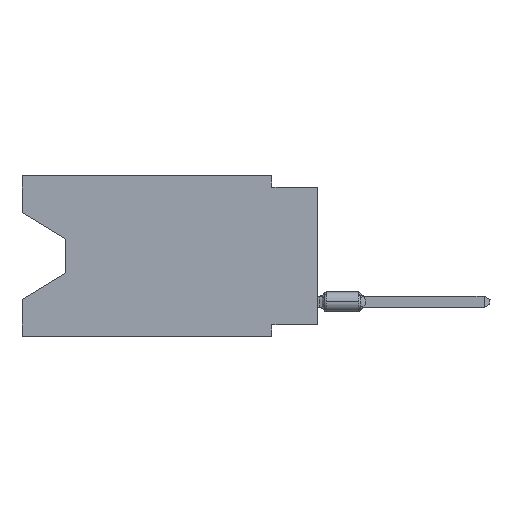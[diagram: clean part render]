
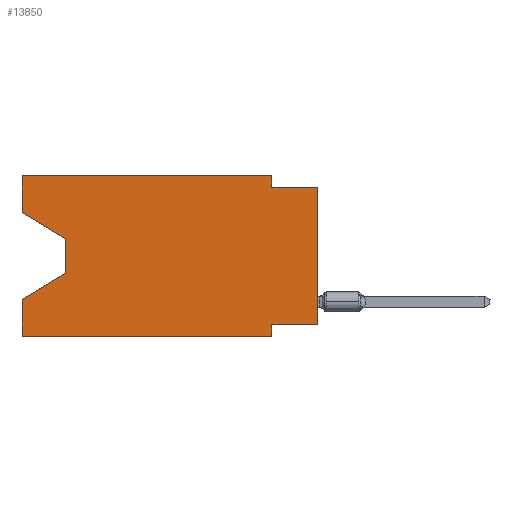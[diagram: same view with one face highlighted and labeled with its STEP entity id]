
A CAD part, left-side view. The second image highlights one B-rep face of the part: STEP entity #13850.
In plain terms, the highlighted planar face has unit normal (-1, 0, 0).
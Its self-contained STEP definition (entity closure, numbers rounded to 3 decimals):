
#352 = VECTOR ( 'NONE', #19690, 1000. ) ;
#1337 = VERTEX_POINT ( 'NONE', #20342 ) ;
#1892 = DIRECTION ( 'NONE',  ( 0., -1., 0. ) ) ;
#2032 = VECTOR ( 'NONE', #56872, 1000. ) ;
#2133 = CARTESIAN_POINT ( 'NONE',  ( 0., 0., -8.255 ) ) ;
#2474 = DIRECTION ( 'NONE',  ( 0., 0.855, -0.519 ) ) ;
#3121 = CARTESIAN_POINT ( 'NONE',  ( 0., 13.97, -5.385 ) ) ;
#4279 = EDGE_CURVE ( 'NONE', #62181, #1337, #60794, .T. ) ;
#5641 = ORIENTED_EDGE ( 'NONE', *, *, #9047, .T. ) ;
#7039 = CARTESIAN_POINT ( 'NONE',  ( 0., 0., 0. ) ) ;
#7942 = CARTESIAN_POINT ( 'NONE',  ( 0., 2.54, -0.635 ) ) ;
#8095 = ORIENTED_EDGE ( 'NONE', *, *, #42171, .F. ) ;
#8271 = ORIENTED_EDGE ( 'NONE', *, *, #28810, .F. ) ;
#8826 = VECTOR ( 'NONE', #18357, 1000. ) ;
#9047 = EDGE_CURVE ( 'NONE', #52611, #43932, #17225, .T. ) ;
#10908 = ORIENTED_EDGE ( 'NONE', *, *, #61993, .F. ) ;
#11304 = VERTEX_POINT ( 'NONE', #34492 ) ;
#11688 = DIRECTION ( 'NONE',  ( 0., -0.855, -0.519 ) ) ;
#13259 = LINE ( 'NONE', #28672, #27764 ) ;
#13850 = ADVANCED_FACE ( 'NONE', ( #31483 ), #57066, .F. ) ;
#14158 = ORIENTED_EDGE ( 'NONE', *, *, #15059, .T. ) ;
#14259 = VERTEX_POINT ( 'NONE', #31395 ) ;
#15059 = EDGE_CURVE ( 'NONE', #62181, #52611, #46918, .T. ) ;
#16546 = EDGE_CURVE ( 'NONE', #31232, #48138, #16653, .T. ) ;
#16595 = CARTESIAN_POINT ( 'NONE',  ( 0., 13.97, -3.505 ) ) ;
#16653 = LINE ( 'NONE', #7039, #27128 ) ;
#17225 = LINE ( 'NONE', #16595, #24915 ) ;
#17438 = DIRECTION ( 'NONE',  ( 0., 0., -1. ) ) ;
#17905 = LINE ( 'NONE', #32003, #44070 ) ;
#18357 = DIRECTION ( 'NONE',  ( 0., -1., 0. ) ) ;
#18675 = LINE ( 'NONE', #58027, #8826 ) ;
#19690 = DIRECTION ( 'NONE',  ( 0., -1., 0. ) ) ;
#20342 = CARTESIAN_POINT ( 'NONE',  ( 0., 16.383, 0. ) ) ;
#21467 = LINE ( 'NONE', #51500, #58059 ) ;
#22354 = CARTESIAN_POINT ( 'NONE',  ( 0., 16.383, -6.852 ) ) ;
#23044 = ORIENTED_EDGE ( 'NONE', *, *, #61592, .F. ) ;
#24915 = VECTOR ( 'NONE', #60155, 1000. ) ;
#26529 = VECTOR ( 'NONE', #50266, 1000. ) ;
#26585 = DIRECTION ( 'NONE',  ( 0., 0., 1. ) ) ;
#26794 = CARTESIAN_POINT ( 'NONE',  ( 0., 16.383, -2.038 ) ) ;
#27128 = VECTOR ( 'NONE', #46400, 1000. ) ;
#27764 = VECTOR ( 'NONE', #17438, 1000. ) ;
#28672 = CARTESIAN_POINT ( 'NONE',  ( 0., 2.54, -8.89 ) ) ;
#28810 = EDGE_CURVE ( 'NONE', #34464, #53646, #17905, .T. ) ;
#30456 = CARTESIAN_POINT ( 'NONE',  ( 0., 16.383, 0. ) ) ;
#31232 = VERTEX_POINT ( 'NONE', #36531 ) ;
#31395 = CARTESIAN_POINT ( 'NONE',  ( 0., 2.54, -8.255 ) ) ;
#31483 = FACE_OUTER_BOUND ( 'NONE', #56777, .T. ) ;
#32003 = CARTESIAN_POINT ( 'NONE',  ( 0., 2.54, 0. ) ) ;
#34364 = CARTESIAN_POINT ( 'NONE',  ( 0., 2.54, 0. ) ) ;
#34464 = VERTEX_POINT ( 'NONE', #34364 ) ;
#34492 = CARTESIAN_POINT ( 'NONE',  ( 0., 2.54, -8.89 ) ) ;
#35527 = LINE ( 'NONE', #40641, #45600 ) ;
#36531 = CARTESIAN_POINT ( 'NONE',  ( 0., 0., -8.255 ) ) ;
#37200 = DIRECTION ( 'NONE',  ( 1., 0., 0. ) ) ;
#37326 = LINE ( 'NONE', #2133, #2032 ) ;
#38382 = EDGE_CURVE ( 'NONE', #54183, #41645, #21467, .T. ) ;
#38821 = CARTESIAN_POINT ( 'NONE',  ( 0., 16.383, -8.89 ) ) ;
#38862 = LINE ( 'NONE', #58086, #352 ) ;
#39522 = CARTESIAN_POINT ( 'NONE',  ( 0., 13.97, -3.505 ) ) ;
#39587 = VECTOR ( 'NONE', #2474, 1000. ) ;
#40066 = ORIENTED_EDGE ( 'NONE', *, *, #4279, .F. ) ;
#40215 = VECTOR ( 'NONE', #11688, 1000. ) ;
#40641 = CARTESIAN_POINT ( 'NONE',  ( 0., 16.383, -8.89 ) ) ;
#41645 = VERTEX_POINT ( 'NONE', #22354 ) ;
#42004 = CARTESIAN_POINT ( 'NONE',  ( 0., 16.383, 0. ) ) ;
#42128 = AXIS2_PLACEMENT_3D ( 'NONE', #42004, #37200, #51305 ) ;
#42171 = EDGE_CURVE ( 'NONE', #1337, #34464, #38862, .T. ) ;
#43932 = VERTEX_POINT ( 'NONE', #52446 ) ;
#44070 = VECTOR ( 'NONE', #46385, 1000. ) ;
#44964 = EDGE_CURVE ( 'NONE', #54183, #11304, #35527, .T. ) ;
#45600 = VECTOR ( 'NONE', #1892, 1000. ) ;
#46385 = DIRECTION ( 'NONE',  ( 0., 0., -1. ) ) ;
#46400 = DIRECTION ( 'NONE',  ( 0., 0., 1. ) ) ;
#46878 = ORIENTED_EDGE ( 'NONE', *, *, #38382, .F. ) ;
#46918 = LINE ( 'NONE', #26794, #40215 ) ;
#48138 = VERTEX_POINT ( 'NONE', #56562 ) ;
#49716 = EDGE_CURVE ( 'NONE', #14259, #11304, #13259, .T. ) ;
#49773 = ORIENTED_EDGE ( 'NONE', *, *, #57723, .T. ) ;
#50266 = DIRECTION ( 'NONE',  ( 0., 0., 1. ) ) ;
#50386 = ORIENTED_EDGE ( 'NONE', *, *, #16546, .T. ) ;
#50832 = LINE ( 'NONE', #3121, #39587 ) ;
#51305 = DIRECTION ( 'NONE',  ( 0., 0., -1. ) ) ;
#51477 = ORIENTED_EDGE ( 'NONE', *, *, #49716, .F. ) ;
#51500 = CARTESIAN_POINT ( 'NONE',  ( 0., 16.383, 0. ) ) ;
#52150 = ORIENTED_EDGE ( 'NONE', *, *, #44964, .T. ) ;
#52446 = CARTESIAN_POINT ( 'NONE',  ( 0., 13.97, -5.385 ) ) ;
#52611 = VERTEX_POINT ( 'NONE', #39522 ) ;
#53646 = VERTEX_POINT ( 'NONE', #7942 ) ;
#53866 = CARTESIAN_POINT ( 'NONE',  ( 0., 16.383, -2.038 ) ) ;
#54183 = VERTEX_POINT ( 'NONE', #38821 ) ;
#56562 = CARTESIAN_POINT ( 'NONE',  ( 0., 0., -0.635 ) ) ;
#56777 = EDGE_LOOP ( 'NONE', ( #14158, #5641, #49773, #46878, #52150, #51477, #23044, #50386, #10908, #8271, #8095, #40066 ) ) ;
#56872 = DIRECTION ( 'NONE',  ( 0., 1., 0. ) ) ;
#57066 = PLANE ( 'NONE',  #42128 ) ;
#57723 = EDGE_CURVE ( 'NONE', #43932, #41645, #50832, .T. ) ;
#58027 = CARTESIAN_POINT ( 'NONE',  ( 0., 0., -0.635 ) ) ;
#58059 = VECTOR ( 'NONE', #26585, 1000. ) ;
#58086 = CARTESIAN_POINT ( 'NONE',  ( 0., 16.383, 0. ) ) ;
#60155 = DIRECTION ( 'NONE',  ( 0., 0., -1. ) ) ;
#60794 = LINE ( 'NONE', #30456, #26529 ) ;
#61592 = EDGE_CURVE ( 'NONE', #31232, #14259, #37326, .T. ) ;
#61993 = EDGE_CURVE ( 'NONE', #53646, #48138, #18675, .T. ) ;
#62181 = VERTEX_POINT ( 'NONE', #53866 ) ;
